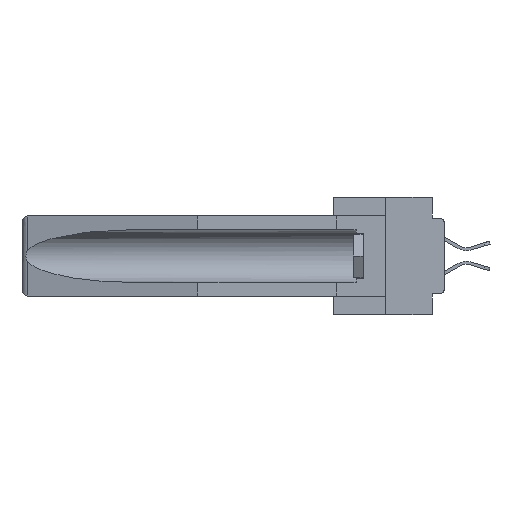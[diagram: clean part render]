
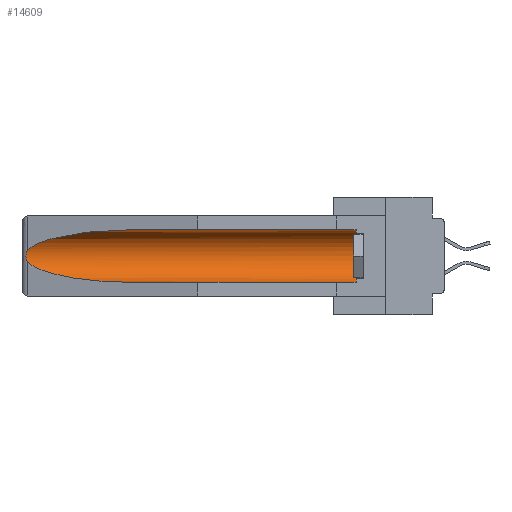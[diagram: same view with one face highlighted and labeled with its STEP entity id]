
A CAD part, left-side view. The second image highlights one B-rep face of the part: STEP entity #14609.
In plain terms, the highlighted cylindrical face has radius 2.857 mm (diameter 5.715 mm), a partial arc.
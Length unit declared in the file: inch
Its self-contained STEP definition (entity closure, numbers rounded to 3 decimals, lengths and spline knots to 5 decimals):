
#522 = DIRECTION ( 'NONE',  ( 0., 1., 0. ) ) ;
#847 = CARTESIAN_POINT ( 'NONE',  ( 0.155, 0.126, -0.059 ) ) ;
#1335 = DIRECTION ( 'NONE',  ( 0., 0., 1. ) ) ;
#2045 = CARTESIAN_POINT ( 'NONE',  ( 0.155, -0.30754, -0.1715 ) ) ;
#2317 = CARTESIAN_POINT ( 'NONE',  ( 0.2675, 1.53308, -0.16763 ) ) ;
#2324 = CARTESIAN_POINT ( 'NONE',  ( 0.155, -0.30754, -0.059 ) ) ;
#3330 = VECTOR ( 'NONE', #522, 39.37008 ) ;
#3546 = ORIENTED_EDGE ( 'NONE', *, *, #30851, .T. ) ;
#3548 = LINE ( 'NONE', #23444, #3330 ) ;
#4133 = EDGE_CURVE ( 'NONE', #27233, #12911, #20933, .T. ) ;
#4248 = CYLINDRICAL_SURFACE ( 'NONE', #26957, 0.1125 ) ;
#4500 = CARTESIAN_POINT ( 'NONE',  ( 0.26597, 1.52961, -0.15275 ) ) ;
#5047 = EDGE_CURVE ( 'NONE', #20119, #15371, #29153, .T. ) ;
#6212 = DIRECTION ( 'NONE',  ( 0., -1., 0. ) ) ;
#6771 = DIRECTION ( 'NONE',  ( 0., 1., 0. ) ) ;
#7259 = ORIENTED_EDGE ( 'NONE', *, *, #5047, .T. ) ;
#7266 = FACE_OUTER_BOUND ( 'NONE', #13277, .T. ) ;
#7305 = CARTESIAN_POINT ( 'NONE',  ( 0.155, 1.07973, -0.284 ) ) ;
#9971 = EDGE_CURVE ( 'NONE', #15371, #20800, #21694, .T. ) ;
#11834 = CARTESIAN_POINT ( 'NONE',  ( 0.26537, 1.52718, -0.14972 ) ) ;
#11877 = CARTESIAN_POINT ( 'NONE',  ( 0.2675, 1.53308, -0.17534 ) ) ;
#12151 = CARTESIAN_POINT ( 'NONE',  ( 0.155, 0.126, -0.284 ) ) ;
#12620 = DIRECTION ( 'NONE',  ( 0., 0., 1. ) ) ;
#12770 = CARTESIAN_POINT ( 'NONE',  ( 0.21114, 1.30732, -0.284 ) ) ;
#12911 = VERTEX_POINT ( 'NONE', #847 ) ;
#13277 = EDGE_LOOP ( 'NONE', ( #7259, #21270, #28129, #32446, #16522, #3546 ) ) ;
#14609 = ADVANCED_FACE ( 'NONE', ( #7266 ), #4248, .F. ) ;
#14894 = DIRECTION ( 'NONE',  ( 0., 1., 0. ) ) ;
#15279 = CARTESIAN_POINT ( 'NONE',  ( 0.25451, 1.48313, -0.09465 ) ) ;
#15371 = VERTEX_POINT ( 'NONE', #11834 ) ;
#15605 = CARTESIAN_POINT ( 'NONE',  ( 0.25451, 1.48313, -0.24835 ) ) ;
#16467 = EDGE_CURVE ( 'NONE', #20800, #17964, #24275, .T. ) ;
#16522 = ORIENTED_EDGE ( 'NONE', *, *, #4133, .T. ) ;
#17050 = CARTESIAN_POINT ( 'NONE',  ( 0.2673, 1.5327, -0.16383 ) ) ;
#17232 = VECTOR ( 'NONE', #14894, 39.37008 ) ;
#17543 = CARTESIAN_POINT ( 'NONE',  ( 0.26597, 1.5296, -0.19026 ) ) ;
#17778 = CARTESIAN_POINT ( 'NONE',  ( 0.155, 1.07973, -0.284 ) ) ;
#17964 = VERTEX_POINT ( 'NONE', #7305 ) ;
#20119 = VERTEX_POINT ( 'NONE', #32879 ) ;
#20800 = VERTEX_POINT ( 'NONE', #28818 ) ;
#20933 = CIRCLE ( 'NONE', #26279, 0.1125 ) ;
#21270 = ORIENTED_EDGE ( 'NONE', *, *, #9971, .T. ) ;
#21694 = B_SPLINE_CURVE_WITH_KNOTS ( 'NONE', 3,
 ( #29898, #4500, #25216, #17050, #2317, #11877, #32562, #32894, #17543, #32400 ),
 .UNSPECIFIED., .F., .F.,
 ( 4, 2, 2, 2, 4 ),
 ( 0., 0.00029, 0.00058, 0.00087, 0.00117 ),
 .UNSPECIFIED. ) ;
#23444 = CARTESIAN_POINT ( 'NONE',  ( 0.155, -0.30754, -0.284 ) ) ;
#24275 =( BOUNDED_CURVE ( )  B_SPLINE_CURVE ( 3, ( #30782, #15605, #12770, #17778 ),
 .UNSPECIFIED., .F., .F. ) 
 B_SPLINE_CURVE_WITH_KNOTS ( ( 4, 4 ),
 ( 0.1948, 1.5708 ),
 .UNSPECIFIED. ) 
 CURVE ( )  GEOMETRIC_REPRESENTATION_ITEM ( )  RATIONAL_B_SPLINE_CURVE ( ( 1., 0.848, 0.848, 1. ) ) 
 REPRESENTATION_ITEM ( '' )  );
#25114 = CARTESIAN_POINT ( 'NONE',  ( 0.155, 1.07973, -0.059 ) ) ;
#25216 = CARTESIAN_POINT ( 'NONE',  ( 0.26654, 1.53092, -0.15636 ) ) ;
#26279 = AXIS2_PLACEMENT_3D ( 'NONE', #32380, #6212, #1335 ) ;
#26957 = AXIS2_PLACEMENT_3D ( 'NONE', #2045, #6771, #12620 ) ;
#27233 = VERTEX_POINT ( 'NONE', #12151 ) ;
#27462 = CARTESIAN_POINT ( 'NONE',  ( 0.21114, 1.30732, -0.059 ) ) ;
#27635 = CARTESIAN_POINT ( 'NONE',  ( 0.26537, 1.52718, -0.14972 ) ) ;
#27911 = EDGE_CURVE ( 'NONE', #27233, #17964, #3548, .T. ) ;
#28129 = ORIENTED_EDGE ( 'NONE', *, *, #16467, .T. ) ;
#28818 = CARTESIAN_POINT ( 'NONE',  ( 0.26537, 1.52718, -0.19328 ) ) ;
#29153 =( BOUNDED_CURVE ( )  B_SPLINE_CURVE ( 3, ( #25114, #27462, #15279, #27635 ),
 .UNSPECIFIED., .F., .F. ) 
 B_SPLINE_CURVE_WITH_KNOTS ( ( 4, 4 ),
 ( 4.71239, 6.08839 ),
 .UNSPECIFIED. ) 
 CURVE ( )  GEOMETRIC_REPRESENTATION_ITEM ( )  RATIONAL_B_SPLINE_CURVE ( ( 1., 0.848, 0.848, 1. ) ) 
 REPRESENTATION_ITEM ( '' )  );
#29898 = CARTESIAN_POINT ( 'NONE',  ( 0.26537, 1.52718, -0.14972 ) ) ;
#30728 = LINE ( 'NONE', #2324, #17232 ) ;
#30782 = CARTESIAN_POINT ( 'NONE',  ( 0.26537, 1.52718, -0.19328 ) ) ;
#30851 = EDGE_CURVE ( 'NONE', #12911, #20119, #30728, .T. ) ;
#32380 = CARTESIAN_POINT ( 'NONE',  ( 0.155, 0.126, -0.1715 ) ) ;
#32400 = CARTESIAN_POINT ( 'NONE',  ( 0.26537, 1.52718, -0.19328 ) ) ;
#32446 = ORIENTED_EDGE ( 'NONE', *, *, #27911, .F. ) ;
#32562 = CARTESIAN_POINT ( 'NONE',  ( 0.2673, 1.53269, -0.17917 ) ) ;
#32879 = CARTESIAN_POINT ( 'NONE',  ( 0.155, 1.07973, -0.059 ) ) ;
#32894 = CARTESIAN_POINT ( 'NONE',  ( 0.26655, 1.53094, -0.18657 ) ) ;
